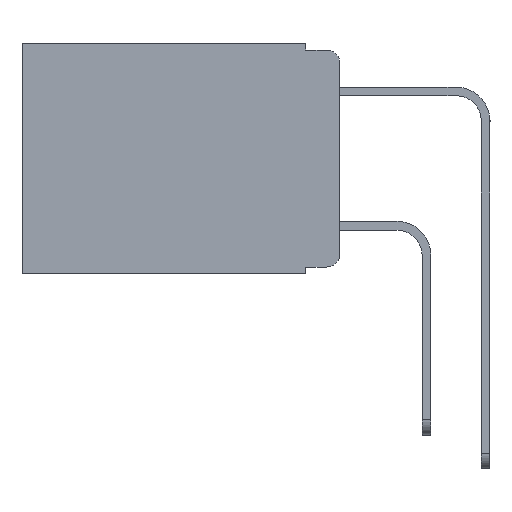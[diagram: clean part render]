
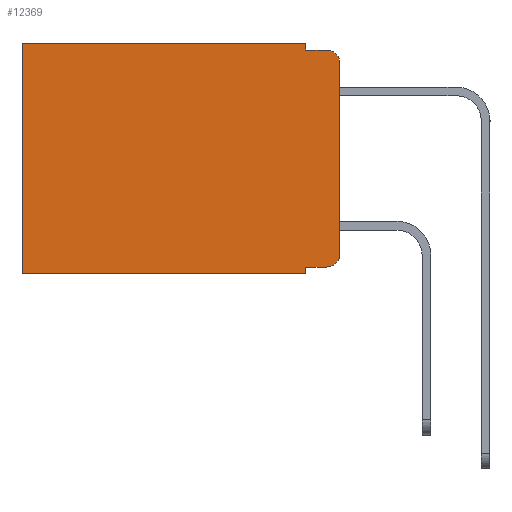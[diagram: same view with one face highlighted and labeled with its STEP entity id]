
A CAD part, left-side view. The second image highlights one B-rep face of the part: STEP entity #12369.
In plain terms, the highlighted planar face has unit normal (-1, 0, 0).
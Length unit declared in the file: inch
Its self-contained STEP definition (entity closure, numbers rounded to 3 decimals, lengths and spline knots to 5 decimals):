
#197 = CARTESIAN_POINT ( 'NONE',  ( 0.298, 0.02, -0.313 ) ) ;
#363 = VERTEX_POINT ( 'NONE', #19194 ) ;
#413 = LINE ( 'NONE', #10922, #10240 ) ;
#1033 = CARTESIAN_POINT ( 'NONE',  ( 0.298, 0., 0. ) ) ;
#1238 = ORIENTED_EDGE ( 'NONE', *, *, #23984, .T. ) ;
#1767 = VERTEX_POINT ( 'NONE', #21694 ) ;
#1917 = LINE ( 'NONE', #23837, #16794 ) ;
#2012 = AXIS2_PLACEMENT_3D ( 'NONE', #19470, #7954, #21401 ) ;
#2035 = LINE ( 'NONE', #1033, #22669 ) ;
#2184 = DIRECTION ( 'NONE',  ( 0., 0., -1. ) ) ;
#2591 = VECTOR ( 'NONE', #14358, 39.37008 ) ;
#3131 = CARTESIAN_POINT ( 'NONE',  ( 0.298, 0.051, 0. ) ) ;
#3153 = AXIS2_PLACEMENT_3D ( 'NONE', #197, #13853, #2184 ) ;
#3215 = DIRECTION ( 'NONE',  ( 0., 0., -1. ) ) ;
#3359 = ORIENTED_EDGE ( 'NONE', *, *, #14153, .F. ) ;
#3998 = ORIENTED_EDGE ( 'NONE', *, *, #18351, .F. ) ;
#4909 = ORIENTED_EDGE ( 'NONE', *, *, #16724, .T. ) ;
#5122 = FACE_OUTER_BOUND ( 'NONE', #18676, .T. ) ;
#5262 = CARTESIAN_POINT ( 'NONE',  ( 0.298, 0.473, -0.343 ) ) ;
#5277 = VERTEX_POINT ( 'NONE', #22314 ) ;
#5972 = VECTOR ( 'NONE', #3215, 39.37008 ) ;
#6417 = ORIENTED_EDGE ( 'NONE', *, *, #17570, .F. ) ;
#6442 = VERTEX_POINT ( 'NONE', #5262 ) ;
#7095 = CARTESIAN_POINT ( 'NONE',  ( 0.298, 0.051, 0. ) ) ;
#7248 = VECTOR ( 'NONE', #14125, 39.37008 ) ;
#7519 = DIRECTION ( 'NONE',  ( 0., 0., -1. ) ) ;
#7954 = DIRECTION ( 'NONE',  ( -1., 0., 0. ) ) ;
#8296 = ORIENTED_EDGE ( 'NONE', *, *, #22812, .T. ) ;
#8637 = VERTEX_POINT ( 'NONE', #24128 ) ;
#10240 = VECTOR ( 'NONE', #11008, 39.37008 ) ;
#10421 = ORIENTED_EDGE ( 'NONE', *, *, #15463, .F. ) ;
#10922 = CARTESIAN_POINT ( 'NONE',  ( 0.298, 0.051, -0.333 ) ) ;
#11008 = DIRECTION ( 'NONE',  ( 0., -1., 0. ) ) ;
#12173 = CARTESIAN_POINT ( 'NONE',  ( 0.298, 0.051, -0.01 ) ) ;
#12264 = VECTOR ( 'NONE', #18219, 39.37008 ) ;
#12369 = ADVANCED_FACE ( 'NONE', ( #5122 ), #15202, .F. ) ;
#12478 = ORIENTED_EDGE ( 'NONE', *, *, #23245, .F. ) ;
#12491 = EDGE_CURVE ( 'NONE', #8637, #16139, #16911, .T. ) ;
#12716 = DIRECTION ( 'NONE',  ( 0., 1., 0. ) ) ;
#13853 = DIRECTION ( 'NONE',  ( -1., 0., 0. ) ) ;
#14034 = VERTEX_POINT ( 'NONE', #24099 ) ;
#14125 = DIRECTION ( 'NONE',  ( 0., -1., 0. ) ) ;
#14153 = EDGE_CURVE ( 'NONE', #16880, #17179, #21998, .T. ) ;
#14251 = DIRECTION ( 'NONE',  ( 0., 0., -1. ) ) ;
#14276 = CARTESIAN_POINT ( 'NONE',  ( 0.298, 0.473, 0. ) ) ;
#14358 = DIRECTION ( 'NONE',  ( 0., 0., -1. ) ) ;
#14471 = CARTESIAN_POINT ( 'NONE',  ( 0.298, 0.02, -0.01 ) ) ;
#14918 = VERTEX_POINT ( 'NONE', #23854 ) ;
#15202 = PLANE ( 'NONE',  #16802 ) ;
#15463 = EDGE_CURVE ( 'NONE', #14034, #1767, #1917, .T. ) ;
#16139 = VERTEX_POINT ( 'NONE', #14471 ) ;
#16282 = CARTESIAN_POINT ( 'NONE',  ( 0.298, 0., -0.343 ) ) ;
#16724 = EDGE_CURVE ( 'NONE', #363, #6442, #18067, .T. ) ;
#16794 = VECTOR ( 'NONE', #14251, 39.37008 ) ;
#16802 = AXIS2_PLACEMENT_3D ( 'NONE', #17113, #19057, #7519 ) ;
#16880 = VERTEX_POINT ( 'NONE', #7095 ) ;
#16911 = CIRCLE ( 'NONE', #2012, 0.02 ) ;
#17113 = CARTESIAN_POINT ( 'NONE',  ( 0.298, 0., 0. ) ) ;
#17179 = VERTEX_POINT ( 'NONE', #21494 ) ;
#17488 = LINE ( 'NONE', #12173, #7248 ) ;
#17570 = EDGE_CURVE ( 'NONE', #8637, #5277, #24676, .T. ) ;
#17994 = LINE ( 'NONE', #16282, #12264 ) ;
#18067 = LINE ( 'NONE', #14276, #2591 ) ;
#18219 = DIRECTION ( 'NONE',  ( 0., 1., 0. ) ) ;
#18351 = EDGE_CURVE ( 'NONE', #1767, #6442, #17994, .T. ) ;
#18676 = EDGE_LOOP ( 'NONE', ( #6417, #22429, #12478, #3359, #8296, #4909, #3998, #10421, #1238, #22480 ) ) ;
#18971 = VECTOR ( 'NONE', #24566, 39.37008 ) ;
#19057 = DIRECTION ( 'NONE',  ( 1., 0., 0. ) ) ;
#19194 = CARTESIAN_POINT ( 'NONE',  ( 0.298, 0.473, 0. ) ) ;
#19470 = CARTESIAN_POINT ( 'NONE',  ( 0.298, 0.02, -0.03 ) ) ;
#20601 = EDGE_CURVE ( 'NONE', #14918, #5277, #23615, .T. ) ;
#21401 = DIRECTION ( 'NONE',  ( 0., 0., -1. ) ) ;
#21494 = CARTESIAN_POINT ( 'NONE',  ( 0.298, 0.051, -0.01 ) ) ;
#21694 = CARTESIAN_POINT ( 'NONE',  ( 0.298, 0.051, -0.343 ) ) ;
#21998 = LINE ( 'NONE', #3131, #5972 ) ;
#22314 = CARTESIAN_POINT ( 'NONE',  ( 0.298, 0., -0.313 ) ) ;
#22429 = ORIENTED_EDGE ( 'NONE', *, *, #12491, .T. ) ;
#22480 = ORIENTED_EDGE ( 'NONE', *, *, #20601, .T. ) ;
#22669 = VECTOR ( 'NONE', #12716, 39.37008 ) ;
#22679 = CARTESIAN_POINT ( 'NONE',  ( 0.298, 0., 0. ) ) ;
#22812 = EDGE_CURVE ( 'NONE', #16880, #363, #2035, .T. ) ;
#23245 = EDGE_CURVE ( 'NONE', #17179, #16139, #17488, .T. ) ;
#23615 = CIRCLE ( 'NONE', #3153, 0.02 ) ;
#23837 = CARTESIAN_POINT ( 'NONE',  ( 0.298, 0.051, 0. ) ) ;
#23854 = CARTESIAN_POINT ( 'NONE',  ( 0.298, 0.02, -0.333 ) ) ;
#23984 = EDGE_CURVE ( 'NONE', #14034, #14918, #413, .T. ) ;
#24099 = CARTESIAN_POINT ( 'NONE',  ( 0.298, 0.051, -0.333 ) ) ;
#24128 = CARTESIAN_POINT ( 'NONE',  ( 0.298, 0., -0.03 ) ) ;
#24566 = DIRECTION ( 'NONE',  ( 0., 0., -1. ) ) ;
#24676 = LINE ( 'NONE', #22679, #18971 ) ;
